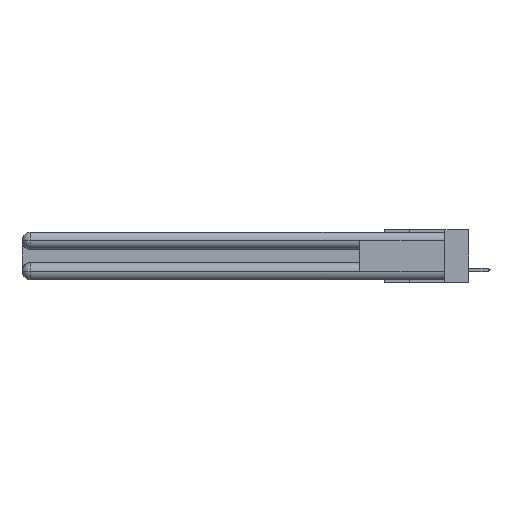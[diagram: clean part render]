
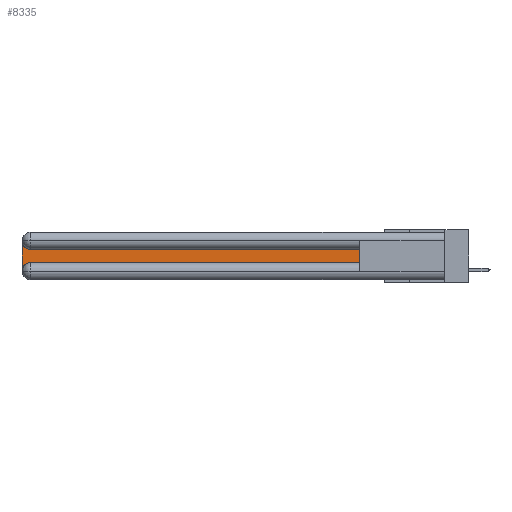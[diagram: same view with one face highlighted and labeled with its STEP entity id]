
A CAD part, left-side view. The second image highlights one B-rep face of the part: STEP entity #8335.
In plain terms, the highlighted planar face has unit normal (-1, 0, 0).
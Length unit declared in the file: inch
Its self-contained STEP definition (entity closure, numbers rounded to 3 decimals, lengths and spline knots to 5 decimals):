
#156 = VERTEX_POINT ( 'NONE', #21129 ) ;
#541 = CARTESIAN_POINT ( 'NONE',  ( 0.075, 0.6, -0.1225 ) ) ;
#1322 = CIRCLE ( 'NONE', #14143, 0.06 ) ;
#2351 = ORIENTED_EDGE ( 'NONE', *, *, #27044, .T. ) ;
#2665 = LINE ( 'NONE', #15873, #5892 ) ;
#2792 = LINE ( 'NONE', #28439, #10039 ) ;
#3421 = CARTESIAN_POINT ( 'NONE',  ( 0.075, 2.94, -0.1225 ) ) ;
#4188 = PLANE ( 'NONE',  #21402 ) ;
#4506 = ORIENTED_EDGE ( 'NONE', *, *, #30243, .T. ) ;
#4507 = CIRCLE ( 'NONE', #16388, 0.06 ) ;
#4955 = EDGE_CURVE ( 'NONE', #156, #15896, #30047, .T. ) ;
#5385 = DIRECTION ( 'NONE',  ( 0., -1., 0. ) ) ;
#5892 = VECTOR ( 'NONE', #10522, 39.37008 ) ;
#5911 = ORIENTED_EDGE ( 'NONE', *, *, #23793, .T. ) ;
#7251 = FACE_OUTER_BOUND ( 'NONE', #15976, .T. ) ;
#7283 = CARTESIAN_POINT ( 'NONE',  ( 0.075, 2.94, -0.2175 ) ) ;
#8335 = ADVANCED_FACE ( 'NONE', ( #7251 ), #4188, .F. ) ;
#9778 = CARTESIAN_POINT ( 'NONE',  ( 0.075, 0.6, -0.2175 ) ) ;
#10039 = VECTOR ( 'NONE', #5385, 39.37008 ) ;
#10046 = CARTESIAN_POINT ( 'NONE',  ( 0.075, 3., -0.0625 ) ) ;
#10522 = DIRECTION ( 'NONE',  ( 0., 0., -1. ) ) ;
#11562 = LINE ( 'NONE', #9778, #25315 ) ;
#11878 = EDGE_CURVE ( 'NONE', #15896, #18636, #1322, .T. ) ;
#12388 = DIRECTION ( 'NONE',  ( 0., 0., 1. ) ) ;
#12429 = CARTESIAN_POINT ( 'NONE',  ( 0.075, 2.94, -0.2775 ) ) ;
#14143 = AXIS2_PLACEMENT_3D ( 'NONE', #25419, #27678, #14825 ) ;
#14151 = DIRECTION ( 'NONE',  ( 0., 0., -1. ) ) ;
#14825 = DIRECTION ( 'NONE',  ( 0., 0., -1. ) ) ;
#15873 = CARTESIAN_POINT ( 'NONE',  ( 0.075, 3., -0.2175 ) ) ;
#15896 = VERTEX_POINT ( 'NONE', #3421 ) ;
#15976 = EDGE_LOOP ( 'NONE', ( #16232, #26062, #4506, #2351, #21368, #5911 ) ) ;
#16232 = ORIENTED_EDGE ( 'NONE', *, *, #4955, .T. ) ;
#16388 = AXIS2_PLACEMENT_3D ( 'NONE', #12429, #17862, #23050 ) ;
#16951 = EDGE_CURVE ( 'NONE', #23804, #17976, #2792, .T. ) ;
#17862 = DIRECTION ( 'NONE',  ( 1., 0., 0. ) ) ;
#17976 = VERTEX_POINT ( 'NONE', #21846 ) ;
#18636 = VERTEX_POINT ( 'NONE', #10046 ) ;
#18934 = DIRECTION ( 'NONE',  ( 0., 1., 0. ) ) ;
#21129 = CARTESIAN_POINT ( 'NONE',  ( 0.075, 0.6, -0.1225 ) ) ;
#21368 = ORIENTED_EDGE ( 'NONE', *, *, #16951, .T. ) ;
#21402 = AXIS2_PLACEMENT_3D ( 'NONE', #24653, #27012, #14151 ) ;
#21846 = CARTESIAN_POINT ( 'NONE',  ( 0.075, 0.6, -0.2175 ) ) ;
#22464 = VERTEX_POINT ( 'NONE', #28972 ) ;
#23050 = DIRECTION ( 'NONE',  ( 0., 0., -1. ) ) ;
#23238 = VECTOR ( 'NONE', #18934, 39.37008 ) ;
#23793 = EDGE_CURVE ( 'NONE', #17976, #156, #11562, .T. ) ;
#23804 = VERTEX_POINT ( 'NONE', #7283 ) ;
#24653 = CARTESIAN_POINT ( 'NONE',  ( 0.075, 3., -0.1225 ) ) ;
#25315 = VECTOR ( 'NONE', #12388, 39.37008 ) ;
#25419 = CARTESIAN_POINT ( 'NONE',  ( 0.075, 2.94, -0.0625 ) ) ;
#26062 = ORIENTED_EDGE ( 'NONE', *, *, #11878, .T. ) ;
#27012 = DIRECTION ( 'NONE',  ( 1., 0., 0. ) ) ;
#27044 = EDGE_CURVE ( 'NONE', #22464, #23804, #4507, .T. ) ;
#27678 = DIRECTION ( 'NONE',  ( 1., 0., 0. ) ) ;
#28439 = CARTESIAN_POINT ( 'NONE',  ( 0.075, 0.6, -0.2175 ) ) ;
#28972 = CARTESIAN_POINT ( 'NONE',  ( 0.075, 3., -0.2775 ) ) ;
#30047 = LINE ( 'NONE', #541, #23238 ) ;
#30243 = EDGE_CURVE ( 'NONE', #18636, #22464, #2665, .T. ) ;
